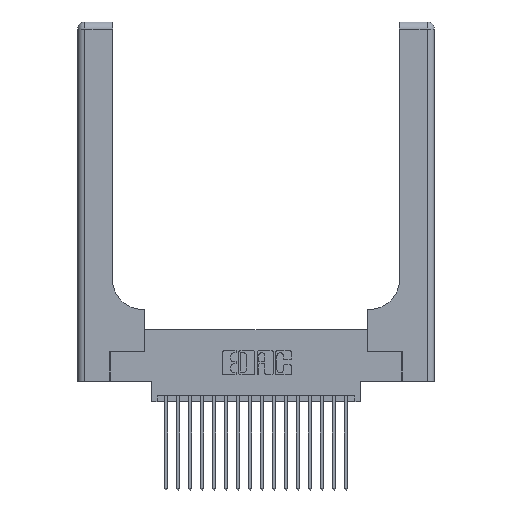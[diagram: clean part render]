
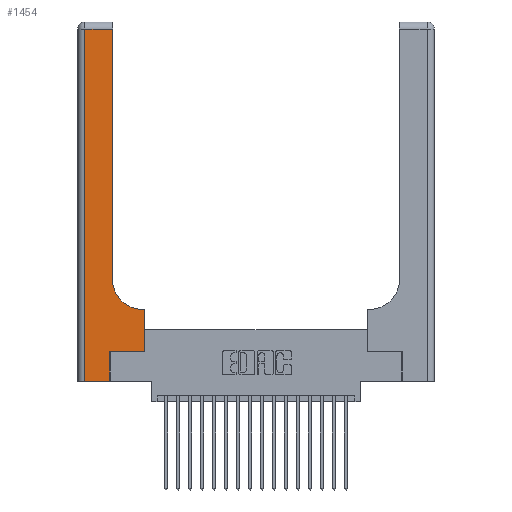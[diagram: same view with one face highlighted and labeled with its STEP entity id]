
A CAD part, top view. The second image highlights one B-rep face of the part: STEP entity #1454.
In plain terms, the highlighted planar face has unit normal (0, 0, 1).
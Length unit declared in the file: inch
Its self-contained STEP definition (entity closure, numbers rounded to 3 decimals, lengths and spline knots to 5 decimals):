
#367 = ORIENTED_EDGE ( 'NONE', *, *, #6393, .T. ) ;
#859 = CARTESIAN_POINT ( 'NONE',  ( 0.269, 0., 0.37 ) ) ;
#890 = DIRECTION ( 'NONE',  ( 0., -1., 0. ) ) ;
#1454 = ADVANCED_FACE ( 'NONE', ( #16460 ), #20228, .F. ) ;
#2506 = DIRECTION ( 'NONE',  ( 1., 0., 0. ) ) ;
#2720 = CARTESIAN_POINT ( 'NONE',  ( 0.269, 0.25, 0.37 ) ) ;
#2757 = CARTESIAN_POINT ( 'NONE',  ( 0.06, 2.94, 0.37 ) ) ;
#2833 = DIRECTION ( 'NONE',  ( -1., 0., 0. ) ) ;
#3385 = ORIENTED_EDGE ( 'NONE', *, *, #17969, .T. ) ;
#3640 = DIRECTION ( 'NONE',  ( 0., 0., -1. ) ) ;
#3652 = EDGE_CURVE ( 'NONE', #14008, #5472, #5742, .T. ) ;
#3711 = DIRECTION ( 'NONE',  ( 0., 1., 0. ) ) ;
#3772 = AXIS2_PLACEMENT_3D ( 'NONE', #13414, #3640, #11973 ) ;
#3779 = CARTESIAN_POINT ( 'NONE',  ( 0.5585, 0.25, 0.37 ) ) ;
#4250 = LINE ( 'NONE', #9355, #8647 ) ;
#4345 = CARTESIAN_POINT ( 'NONE',  ( 0.2915, 2.94, 0.37 ) ) ;
#4381 = LINE ( 'NONE', #20134, #17811 ) ;
#4592 = VECTOR ( 'NONE', #890, 39.37008 ) ;
#4616 = VECTOR ( 'NONE', #11847, 39.37008 ) ;
#4882 = CARTESIAN_POINT ( 'NONE',  ( 0.06, 0., 0.37 ) ) ;
#5142 = EDGE_CURVE ( 'NONE', #5472, #15919, #4381, .T. ) ;
#5295 = CARTESIAN_POINT ( 'NONE',  ( 0.2915, 0.6, 0.37 ) ) ;
#5325 = DIRECTION ( 'NONE',  ( 0., 1., 0. ) ) ;
#5399 = ORIENTED_EDGE ( 'NONE', *, *, #6882, .T. ) ;
#5472 = VERTEX_POINT ( 'NONE', #859 ) ;
#5742 = LINE ( 'NONE', #15643, #7040 ) ;
#5809 = EDGE_CURVE ( 'NONE', #14514, #16705, #11075, .T. ) ;
#6206 = DIRECTION ( 'NONE',  ( 0., 1., 0. ) ) ;
#6393 = EDGE_CURVE ( 'NONE', #16705, #17745, #9806, .T. ) ;
#6505 = VERTEX_POINT ( 'NONE', #3779 ) ;
#6588 = DIRECTION ( 'NONE',  ( 0., 0., -1. ) ) ;
#6882 = EDGE_CURVE ( 'NONE', #6505, #14514, #8472, .T. ) ;
#7040 = VECTOR ( 'NONE', #7105, 39.37008 ) ;
#7105 = DIRECTION ( 'NONE',  ( 1., 0., 0. ) ) ;
#7879 = EDGE_CURVE ( 'NONE', #15919, #6505, #17982, .T. ) ;
#7901 = ORIENTED_EDGE ( 'NONE', *, *, #5809, .T. ) ;
#8249 = ORIENTED_EDGE ( 'NONE', *, *, #18406, .T. ) ;
#8269 = DIRECTION ( 'NONE',  ( 1., 0., 0. ) ) ;
#8472 = LINE ( 'NONE', #14260, #10285 ) ;
#8647 = VECTOR ( 'NONE', #2833, 39.37008 ) ;
#8664 = CARTESIAN_POINT ( 'NONE',  ( 0.5415, 0.6, 0.37 ) ) ;
#9141 = CARTESIAN_POINT ( 'NONE',  ( 0.06, 3., 0.37 ) ) ;
#9206 = ORIENTED_EDGE ( 'NONE', *, *, #7879, .T. ) ;
#9355 = CARTESIAN_POINT ( 'NONE',  ( 0., 2.94, 0.37 ) ) ;
#9806 = CIRCLE ( 'NONE', #10498, 0.25 ) ;
#10285 = VECTOR ( 'NONE', #6206, 39.37008 ) ;
#10498 = AXIS2_PLACEMENT_3D ( 'NONE', #11753, #6588, #8269 ) ;
#10659 = ORIENTED_EDGE ( 'NONE', *, *, #16540, .T. ) ;
#11067 = VECTOR ( 'NONE', #3711, 39.37008 ) ;
#11075 = LINE ( 'NONE', #5295, #4616 ) ;
#11215 = EDGE_LOOP ( 'NONE', ( #3385, #10659, #8249, #11249, #11608, #9206, #5399, #7901, #367 ) ) ;
#11249 = ORIENTED_EDGE ( 'NONE', *, *, #3652, .T. ) ;
#11608 = ORIENTED_EDGE ( 'NONE', *, *, #5142, .T. ) ;
#11753 = CARTESIAN_POINT ( 'NONE',  ( 0.5415, 0.85, 0.37 ) ) ;
#11762 = CARTESIAN_POINT ( 'NONE',  ( 0.2915, 3., 0.37 ) ) ;
#11847 = DIRECTION ( 'NONE',  ( -1., 0., 0. ) ) ;
#11973 = DIRECTION ( 'NONE',  ( -1., 0., 0. ) ) ;
#13414 = CARTESIAN_POINT ( 'NONE',  ( 0., 3., 0.37 ) ) ;
#13596 = VECTOR ( 'NONE', #2506, 39.37008 ) ;
#14008 = VERTEX_POINT ( 'NONE', #4882 ) ;
#14260 = CARTESIAN_POINT ( 'NONE',  ( 0.5585, 0.25, 0.37 ) ) ;
#14514 = VERTEX_POINT ( 'NONE', #18643 ) ;
#15208 = LINE ( 'NONE', #11762, #11067 ) ;
#15636 = CARTESIAN_POINT ( 'NONE',  ( 0.269, 0.25, 0.37 ) ) ;
#15643 = CARTESIAN_POINT ( 'NONE',  ( 0., 0., 0.37 ) ) ;
#15919 = VERTEX_POINT ( 'NONE', #15636 ) ;
#16391 = VERTEX_POINT ( 'NONE', #2757 ) ;
#16460 = FACE_OUTER_BOUND ( 'NONE', #11215, .T. ) ;
#16463 = LINE ( 'NONE', #9141, #4592 ) ;
#16540 = EDGE_CURVE ( 'NONE', #20535, #16391, #4250, .T. ) ;
#16705 = VERTEX_POINT ( 'NONE', #8664 ) ;
#17745 = VERTEX_POINT ( 'NONE', #17814 ) ;
#17811 = VECTOR ( 'NONE', #5325, 39.37008 ) ;
#17814 = CARTESIAN_POINT ( 'NONE',  ( 0.2915, 0.85, 0.37 ) ) ;
#17969 = EDGE_CURVE ( 'NONE', #17745, #20535, #15208, .T. ) ;
#17982 = LINE ( 'NONE', #2720, #13596 ) ;
#18406 = EDGE_CURVE ( 'NONE', #16391, #14008, #16463, .T. ) ;
#18643 = CARTESIAN_POINT ( 'NONE',  ( 0.5585, 0.6, 0.37 ) ) ;
#20134 = CARTESIAN_POINT ( 'NONE',  ( 0.269, 0., 0.37 ) ) ;
#20228 = PLANE ( 'NONE',  #3772 ) ;
#20535 = VERTEX_POINT ( 'NONE', #4345 ) ;
